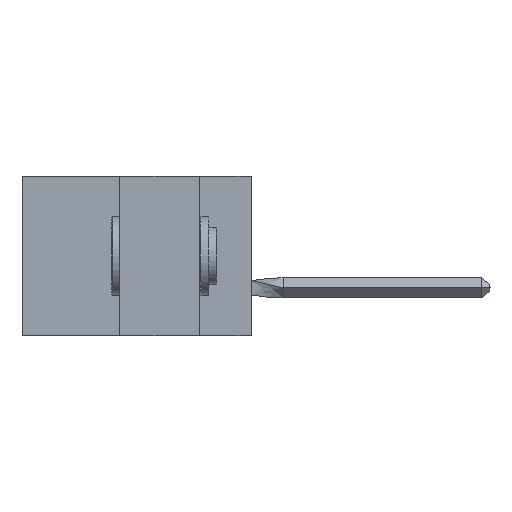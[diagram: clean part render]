
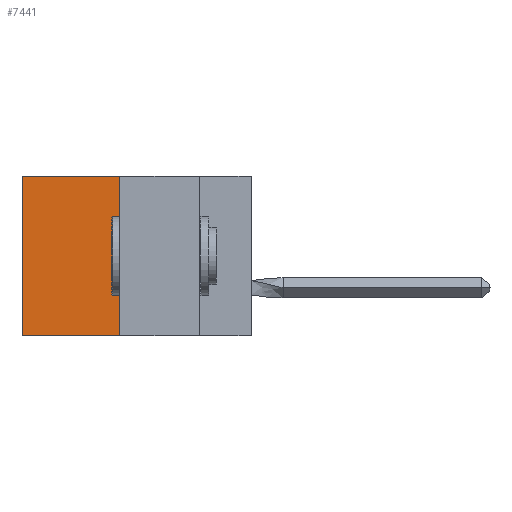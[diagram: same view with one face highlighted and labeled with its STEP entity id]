
A CAD part, left-side view. The second image highlights one B-rep face of the part: STEP entity #7441.
In plain terms, the highlighted planar face has unit normal (-1, 0, 0).
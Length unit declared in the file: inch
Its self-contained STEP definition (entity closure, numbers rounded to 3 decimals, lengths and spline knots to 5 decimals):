
#232 = DIRECTION ( 'NONE',  ( 1., 0., 0. ) ) ;
#672 = DIRECTION ( 'NONE',  ( 0., 1., 0. ) ) ;
#1143 = LINE ( 'NONE', #12773, #26836 ) ;
#2382 = CARTESIAN_POINT ( 'NONE',  ( 0.305, 0.72, -0.5 ) ) ;
#3847 = VERTEX_POINT ( 'NONE', #12905 ) ;
#4057 = DIRECTION ( 'NONE',  ( 0., 0., -1. ) ) ;
#7441 = ADVANCED_FACE ( 'NONE', ( #18536 ), #19417, .F. ) ;
#7849 = VECTOR ( 'NONE', #4057, 39.37008 ) ;
#9795 = EDGE_CURVE ( 'NONE', #12046, #3847, #20239, .T. ) ;
#12046 = VERTEX_POINT ( 'NONE', #12924 ) ;
#12773 = CARTESIAN_POINT ( 'NONE',  ( 0.305, 0.413, -0.5 ) ) ;
#12846 = DIRECTION ( 'NONE',  ( 0., 0., -1. ) ) ;
#12905 = CARTESIAN_POINT ( 'NONE',  ( 0.305, 0.72, 0. ) ) ;
#12924 = CARTESIAN_POINT ( 'NONE',  ( 0.305, 0.413, 0. ) ) ;
#13346 = EDGE_LOOP ( 'NONE', ( #18985, #14772, #19455, #18370 ) ) ;
#13813 = VECTOR ( 'NONE', #12846, 39.37008 ) ;
#14182 = LINE ( 'NONE', #27740, #13813 ) ;
#14772 = ORIENTED_EDGE ( 'NONE', *, *, #19059, .F. ) ;
#15159 = CARTESIAN_POINT ( 'NONE',  ( 0.305, 0.413, -0.5 ) ) ;
#15607 = AXIS2_PLACEMENT_3D ( 'NONE', #15159, #232, #22462 ) ;
#16624 = CARTESIAN_POINT ( 'NONE',  ( 0.305, 0.413, 0. ) ) ;
#18370 = ORIENTED_EDGE ( 'NONE', *, *, #9795, .T. ) ;
#18536 = FACE_OUTER_BOUND ( 'NONE', #13346, .T. ) ;
#18985 = ORIENTED_EDGE ( 'NONE', *, *, #31104, .T. ) ;
#19059 = EDGE_CURVE ( 'NONE', #25856, #26749, #1143, .T. ) ;
#19417 = PLANE ( 'NONE',  #15607 ) ;
#19455 = ORIENTED_EDGE ( 'NONE', *, *, #29590, .F. ) ;
#20239 = LINE ( 'NONE', #16624, #21823 ) ;
#21823 = VECTOR ( 'NONE', #29132, 39.37008 ) ;
#22233 = LINE ( 'NONE', #26484, #7849 ) ;
#22462 = DIRECTION ( 'NONE',  ( 0., 0., -1. ) ) ;
#25856 = VERTEX_POINT ( 'NONE', #28130 ) ;
#26484 = CARTESIAN_POINT ( 'NONE',  ( 0.305, 0.72, -0.5 ) ) ;
#26749 = VERTEX_POINT ( 'NONE', #2382 ) ;
#26836 = VECTOR ( 'NONE', #672, 39.37008 ) ;
#27740 = CARTESIAN_POINT ( 'NONE',  ( 0.305, 0.413, -0.5 ) ) ;
#28130 = CARTESIAN_POINT ( 'NONE',  ( 0.305, 0.413, -0.5 ) ) ;
#29132 = DIRECTION ( 'NONE',  ( 0., 1., 0. ) ) ;
#29590 = EDGE_CURVE ( 'NONE', #12046, #25856, #14182, .T. ) ;
#31104 = EDGE_CURVE ( 'NONE', #3847, #26749, #22233, .T. ) ;
